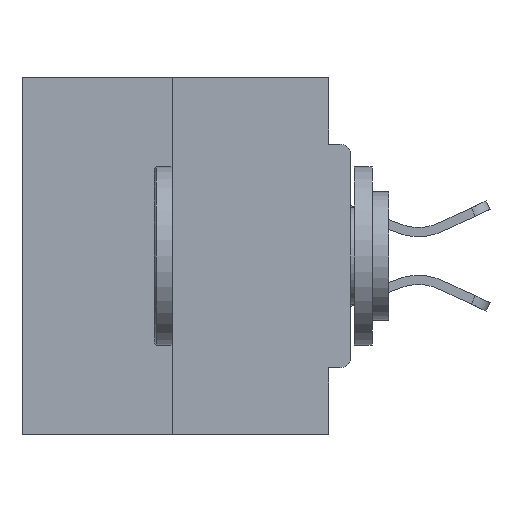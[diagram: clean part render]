
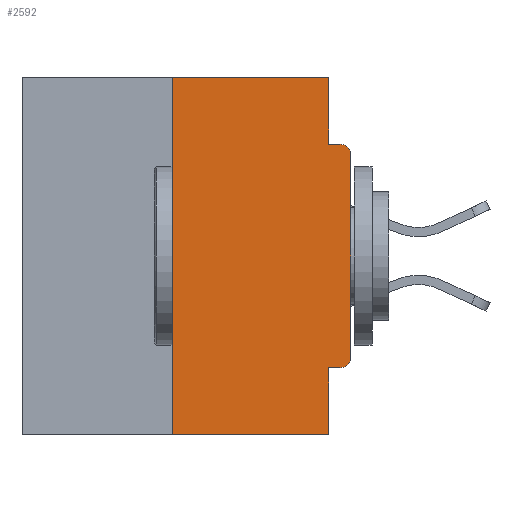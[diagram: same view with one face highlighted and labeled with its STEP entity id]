
A CAD part, left-side view. The second image highlights one B-rep face of the part: STEP entity #2592.
In plain terms, the highlighted planar face has unit normal (-1, 0, 0).
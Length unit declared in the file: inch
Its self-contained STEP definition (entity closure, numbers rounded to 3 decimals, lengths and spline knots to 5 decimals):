
#130 = DIRECTION ( 'NONE',  ( 0., 0., -1. ) ) ;
#173 = LINE ( 'NONE', #1698, #22078 ) ;
#1259 = DIRECTION ( 'NONE',  ( -1., 0., 0. ) ) ;
#1698 = CARTESIAN_POINT ( 'NONE',  ( 0., 0.46, -0.5 ) ) ;
#2479 = ORIENTED_EDGE ( 'NONE', *, *, #27586, .F. ) ;
#2592 = ADVANCED_FACE ( 'NONE', ( #13579 ), #25644, .F. ) ;
#2699 = VECTOR ( 'NONE', #30026, 39.37008 ) ;
#3748 = LINE ( 'NONE', #7232, #31097 ) ;
#4106 = CARTESIAN_POINT ( 'NONE',  ( 0., 0.015, -0.1085 ) ) ;
#4275 = LINE ( 'NONE', #34904, #11797 ) ;
#4955 = CARTESIAN_POINT ( 'NONE',  ( 0., 0., -0.3915 ) ) ;
#5851 = DIRECTION ( 'NONE',  ( 1., 0., 0. ) ) ;
#6159 = DIRECTION ( 'NONE',  ( 0., 0., 1. ) ) ;
#6311 = DIRECTION ( 'NONE',  ( -1., 0., 0. ) ) ;
#6905 = EDGE_CURVE ( 'NONE', #25752, #36670, #173, .T. ) ;
#6996 = DIRECTION ( 'NONE',  ( 0., 0., -1. ) ) ;
#7232 = CARTESIAN_POINT ( 'NONE',  ( 0., 0.031, 0. ) ) ;
#7450 = VERTEX_POINT ( 'NONE', #15681 ) ;
#7765 = CIRCLE ( 'NONE', #20211, 0.015 ) ;
#8473 = LINE ( 'NONE', #23664, #10240 ) ;
#8891 = VECTOR ( 'NONE', #33169, 39.37008 ) ;
#8955 = CARTESIAN_POINT ( 'NONE',  ( 0., 0.031, -0.5 ) ) ;
#9323 = CARTESIAN_POINT ( 'NONE',  ( 0., 0.015, -0.4065 ) ) ;
#9444 = ORIENTED_EDGE ( 'NONE', *, *, #27892, .F. ) ;
#9837 = VERTEX_POINT ( 'NONE', #24269 ) ;
#10240 = VECTOR ( 'NONE', #15346, 39.37008 ) ;
#10532 = EDGE_CURVE ( 'NONE', #25752, #7450, #4275, .T. ) ;
#11228 = CARTESIAN_POINT ( 'NONE',  ( 0., 0.031, -0.0935 ) ) ;
#11797 = VECTOR ( 'NONE', #6159, 39.37008 ) ;
#13306 = ORIENTED_EDGE ( 'NONE', *, *, #10532, .F. ) ;
#13579 = FACE_OUTER_BOUND ( 'NONE', #30206, .T. ) ;
#14681 = CARTESIAN_POINT ( 'NONE',  ( 0., 0., 0. ) ) ;
#15041 = DIRECTION ( 'NONE',  ( 0., 0., -1. ) ) ;
#15230 = VERTEX_POINT ( 'NONE', #28172 ) ;
#15346 = DIRECTION ( 'NONE',  ( 0., -1., 0. ) ) ;
#15433 = CARTESIAN_POINT ( 'NONE',  ( 0., 0.031, -0.5 ) ) ;
#15485 = EDGE_CURVE ( 'NONE', #34595, #18156, #3748, .T. ) ;
#15493 = EDGE_CURVE ( 'NONE', #9837, #17571, #7765, .T. ) ;
#15681 = CARTESIAN_POINT ( 'NONE',  ( 0., 0.25, 0. ) ) ;
#16959 = ORIENTED_EDGE ( 'NONE', *, *, #20461, .T. ) ;
#17372 = ORIENTED_EDGE ( 'NONE', *, *, #31401, .F. ) ;
#17571 = VERTEX_POINT ( 'NONE', #25158 ) ;
#18156 = VERTEX_POINT ( 'NONE', #11228 ) ;
#18499 = DIRECTION ( 'NONE',  ( 0., 0., -1. ) ) ;
#20211 = AXIS2_PLACEMENT_3D ( 'NONE', #4106, #1259, #6996 ) ;
#20461 = EDGE_CURVE ( 'NONE', #25003, #25344, #30235, .T. ) ;
#20840 = EDGE_CURVE ( 'NONE', #25344, #9837, #36145, .T. ) ;
#21139 = CARTESIAN_POINT ( 'NONE',  ( 0., 0., -0.0935 ) ) ;
#21736 = VECTOR ( 'NONE', #36998, 39.37008 ) ;
#22078 = VECTOR ( 'NONE', #33249, 39.37008 ) ;
#22103 = ORIENTED_EDGE ( 'NONE', *, *, #26683, .F. ) ;
#22184 = AXIS2_PLACEMENT_3D ( 'NONE', #31908, #5851, #130 ) ;
#23251 = LINE ( 'NONE', #23775, #8891 ) ;
#23664 = CARTESIAN_POINT ( 'NONE',  ( 0., 0.46, 0. ) ) ;
#23775 = CARTESIAN_POINT ( 'NONE',  ( 0., 0., -0.4065 ) ) ;
#24269 = CARTESIAN_POINT ( 'NONE',  ( 0., 0., -0.1085 ) ) ;
#25003 = VERTEX_POINT ( 'NONE', #9323 ) ;
#25158 = CARTESIAN_POINT ( 'NONE',  ( 0., 0.015, -0.0935 ) ) ;
#25162 = LINE ( 'NONE', #8955, #26491 ) ;
#25344 = VERTEX_POINT ( 'NONE', #4955 ) ;
#25644 = PLANE ( 'NONE',  #22184 ) ;
#25752 = VERTEX_POINT ( 'NONE', #33230 ) ;
#26026 = CARTESIAN_POINT ( 'NONE',  ( 0., 0.031, 0. ) ) ;
#26491 = VECTOR ( 'NONE', #15041, 39.37008 ) ;
#26683 = EDGE_CURVE ( 'NONE', #15230, #36670, #25162, .T. ) ;
#27315 = LINE ( 'NONE', #21139, #2699 ) ;
#27586 = EDGE_CURVE ( 'NONE', #7450, #34595, #8473, .T. ) ;
#27892 = EDGE_CURVE ( 'NONE', #25003, #15230, #23251, .T. ) ;
#28172 = CARTESIAN_POINT ( 'NONE',  ( 0., 0.031, -0.4065 ) ) ;
#28290 = ORIENTED_EDGE ( 'NONE', *, *, #20840, .T. ) ;
#30026 = DIRECTION ( 'NONE',  ( 0., -1., 0. ) ) ;
#30206 = EDGE_LOOP ( 'NONE', ( #2479, #13306, #30616, #22103, #9444, #16959, #28290, #34872, #17372, #32380 ) ) ;
#30235 = CIRCLE ( 'NONE', #31656, 0.015 ) ;
#30616 = ORIENTED_EDGE ( 'NONE', *, *, #6905, .T. ) ;
#31097 = VECTOR ( 'NONE', #18499, 39.37008 ) ;
#31401 = EDGE_CURVE ( 'NONE', #18156, #17571, #27315, .T. ) ;
#31656 = AXIS2_PLACEMENT_3D ( 'NONE', #32513, #6311, #35307 ) ;
#31908 = CARTESIAN_POINT ( 'NONE',  ( 0., 0.46, 0. ) ) ;
#32380 = ORIENTED_EDGE ( 'NONE', *, *, #15485, .F. ) ;
#32513 = CARTESIAN_POINT ( 'NONE',  ( 0., 0.015, -0.3915 ) ) ;
#33169 = DIRECTION ( 'NONE',  ( 0., 1., 0. ) ) ;
#33230 = CARTESIAN_POINT ( 'NONE',  ( 0., 0.25, -0.5 ) ) ;
#33249 = DIRECTION ( 'NONE',  ( 0., -1., 0. ) ) ;
#34595 = VERTEX_POINT ( 'NONE', #26026 ) ;
#34872 = ORIENTED_EDGE ( 'NONE', *, *, #15493, .T. ) ;
#34904 = CARTESIAN_POINT ( 'NONE',  ( 0., 0.25, 0. ) ) ;
#35307 = DIRECTION ( 'NONE',  ( 0., 0., -1. ) ) ;
#36145 = LINE ( 'NONE', #14681, #21736 ) ;
#36670 = VERTEX_POINT ( 'NONE', #15433 ) ;
#36998 = DIRECTION ( 'NONE',  ( 0., 0., 1. ) ) ;
